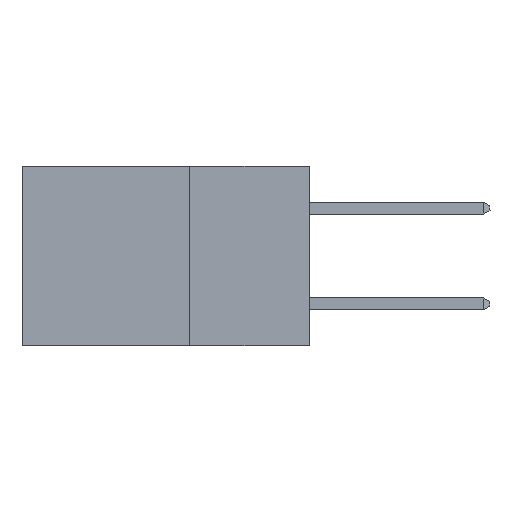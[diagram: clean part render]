
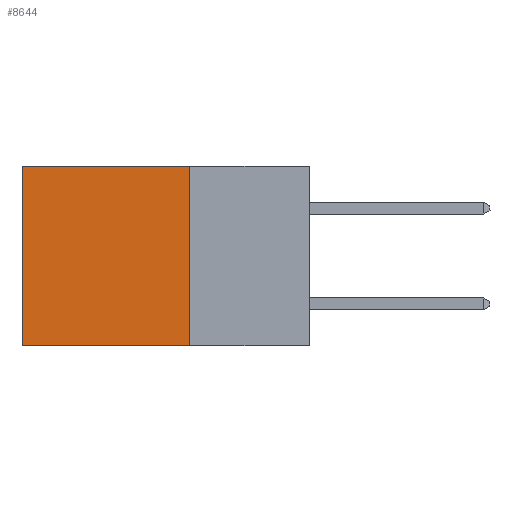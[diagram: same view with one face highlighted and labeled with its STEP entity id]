
A CAD part, left-side view. The second image highlights one B-rep face of the part: STEP entity #8644.
In plain terms, the highlighted planar face has unit normal (-1, 0, 0).
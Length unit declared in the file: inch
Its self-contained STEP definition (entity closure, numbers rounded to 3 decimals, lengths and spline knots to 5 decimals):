
#25 = VERTEX_POINT ( 'NONE', #6334 ) ;
#407 = CARTESIAN_POINT ( 'NONE',  ( 0.2875, 0.6, 0. ) ) ;
#479 = CARTESIAN_POINT ( 'NONE',  ( 0.2875, 0.6, -0.375 ) ) ;
#485 = FACE_OUTER_BOUND ( 'NONE', #1080, .T. ) ;
#598 = LINE ( 'NONE', #9345, #8334 ) ;
#901 = EDGE_CURVE ( 'NONE', #6853, #8995, #6483, .T. ) ;
#1080 = EDGE_LOOP ( 'NONE', ( #5917, #3558, #6138, #6288 ) ) ;
#1607 = CARTESIAN_POINT ( 'NONE',  ( 0.2875, 0.25, -0.375 ) ) ;
#1632 = DIRECTION ( 'NONE',  ( 1., 0., 0. ) ) ;
#1948 = LINE ( 'NONE', #4422, #9736 ) ;
#3125 = CARTESIAN_POINT ( 'NONE',  ( 0.2875, 0.6, -0.375 ) ) ;
#3558 = ORIENTED_EDGE ( 'NONE', *, *, #9409, .F. ) ;
#3599 = DIRECTION ( 'NONE',  ( 0., 0., -1. ) ) ;
#4004 = AXIS2_PLACEMENT_3D ( 'NONE', #6170, #1632, #7663 ) ;
#4007 = VERTEX_POINT ( 'NONE', #1607 ) ;
#4065 = DIRECTION ( 'NONE',  ( 0., 1., 0. ) ) ;
#4422 = CARTESIAN_POINT ( 'NONE',  ( 0.2875, 0.25, -0.375 ) ) ;
#4460 = EDGE_CURVE ( 'NONE', #25, #4007, #1948, .T. ) ;
#4483 = VECTOR ( 'NONE', #6084, 39.37008 ) ;
#5080 = VECTOR ( 'NONE', #7428, 39.37008 ) ;
#5917 = ORIENTED_EDGE ( 'NONE', *, *, #901, .T. ) ;
#6084 = DIRECTION ( 'NONE',  ( 0., 0., -1. ) ) ;
#6138 = ORIENTED_EDGE ( 'NONE', *, *, #4460, .F. ) ;
#6170 = CARTESIAN_POINT ( 'NONE',  ( 0.2875, 0.25, -0.375 ) ) ;
#6288 = ORIENTED_EDGE ( 'NONE', *, *, #6314, .T. ) ;
#6314 = EDGE_CURVE ( 'NONE', #25, #6853, #6598, .T. ) ;
#6334 = CARTESIAN_POINT ( 'NONE',  ( 0.2875, 0.25, 0. ) ) ;
#6483 = LINE ( 'NONE', #3125, #4483 ) ;
#6587 = CARTESIAN_POINT ( 'NONE',  ( 0.2875, 0.25, 0. ) ) ;
#6598 = LINE ( 'NONE', #6587, #5080 ) ;
#6853 = VERTEX_POINT ( 'NONE', #407 ) ;
#7428 = DIRECTION ( 'NONE',  ( 0., 1., 0. ) ) ;
#7663 = DIRECTION ( 'NONE',  ( 0., 0., -1. ) ) ;
#8334 = VECTOR ( 'NONE', #4065, 39.37008 ) ;
#8644 = ADVANCED_FACE ( 'NONE', ( #485 ), #9260, .F. ) ;
#8995 = VERTEX_POINT ( 'NONE', #479 ) ;
#9260 = PLANE ( 'NONE',  #4004 ) ;
#9345 = CARTESIAN_POINT ( 'NONE',  ( 0.2875, 0.25, -0.375 ) ) ;
#9409 = EDGE_CURVE ( 'NONE', #4007, #8995, #598, .T. ) ;
#9736 = VECTOR ( 'NONE', #3599, 39.37008 ) ;
